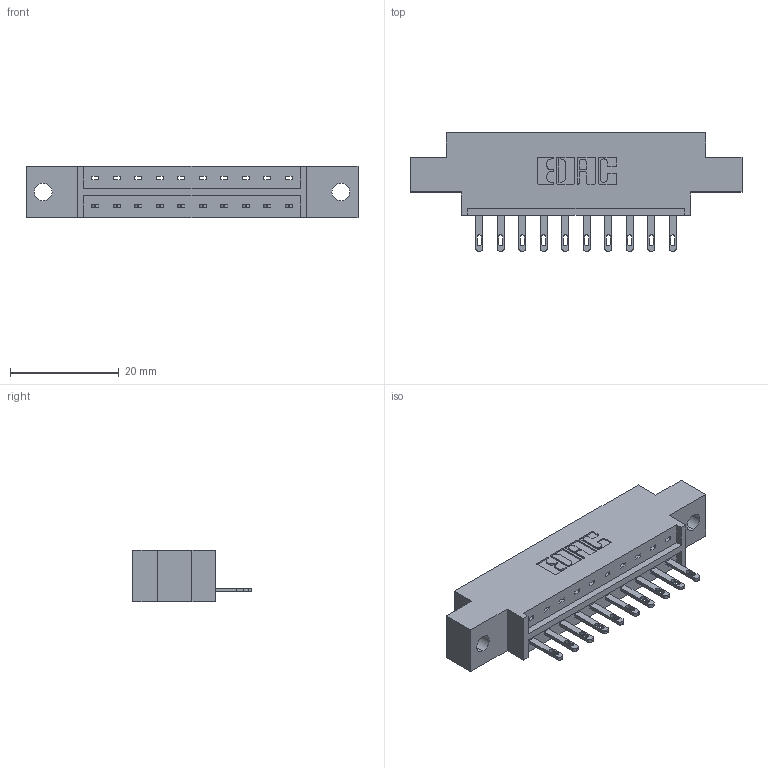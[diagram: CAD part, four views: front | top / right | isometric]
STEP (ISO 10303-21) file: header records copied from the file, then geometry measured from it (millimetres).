
FILE_DESCRIPTION (( 'STEP AP203' ), '1' );
FILE_NAME ('833-010-500-602.STEP', '2020-05-30T18:00:31', ( '' ), ( '' ), 'SwSTEP 2.0', 'SolidWorks 2020', '' );
FILE_SCHEMA (( 'CONFIG_CONTROL_DESIGN' ));
Length unit declared in the file: inch
Products named in the file (3): 833 Part_Offset - .128 Dia; 833-010-500-602; 345-292-001_345-293-100
Assembly tree (11 placements, depth 2):
  833-010-500-602
    833 Part_Offset - .128 Dia
    345-292-001_345-293-100  x10
Bounding box: 61.16 x 21.85 x 9.4 mm (x, y, z)
Volume: 5621.3 mm3; surface area: 5822.6 mm2
Topology: 11 solids, 11 shells, 658 faces, 2003 edges, 1334 vertices
Faces by surface type: plane 434, cylinder 224
Entity records: 10317 total; most frequent: CARTESIAN_POINT 1792, ORIENTED_EDGE 1738, DIRECTION 1577, EDGE_CURVE 869, LINE 737, VECTOR 737, VERTEX_POINT 578, AXIS2_PLACEMENT_3D 420
